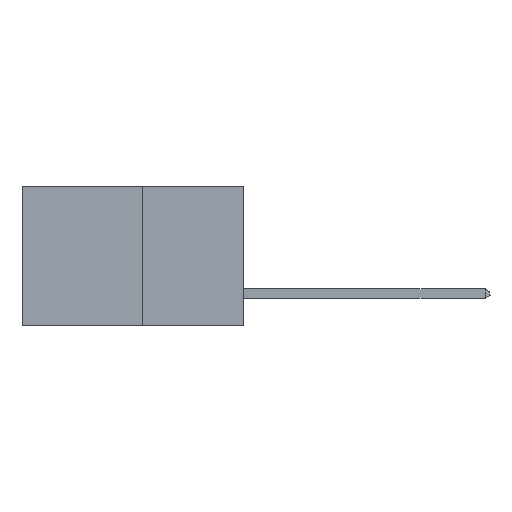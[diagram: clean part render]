
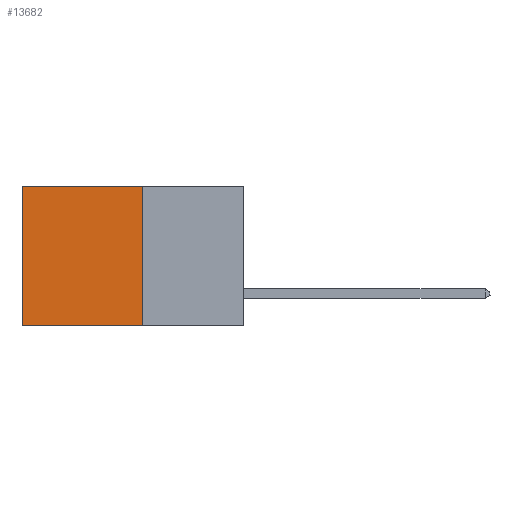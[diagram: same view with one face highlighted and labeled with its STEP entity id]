
A CAD part, left-side view. The second image highlights one B-rep face of the part: STEP entity #13682.
In plain terms, the highlighted planar face has unit normal (-1, 0, 0).
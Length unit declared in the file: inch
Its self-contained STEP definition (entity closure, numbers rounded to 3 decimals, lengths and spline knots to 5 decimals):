
#685 = CARTESIAN_POINT ( 'NONE',  ( 0.277, 0.59, -0.37 ) ) ;
#1333 = VERTEX_POINT ( 'NONE', #685 ) ;
#1390 = EDGE_CURVE ( 'NONE', #10217, #12038, #2702, .T. ) ;
#1473 = AXIS2_PLACEMENT_3D ( 'NONE', #10987, #12049, #5614 ) ;
#1802 = CARTESIAN_POINT ( 'NONE',  ( 0.277, 0.27, -0.37 ) ) ;
#1866 = ORIENTED_EDGE ( 'NONE', *, *, #10497, .T. ) ;
#2213 = ORIENTED_EDGE ( 'NONE', *, *, #12834, .F. ) ;
#2236 = DIRECTION ( 'NONE',  ( 0., 0., -1. ) ) ;
#2417 = CARTESIAN_POINT ( 'NONE',  ( 0.277, 0.27, 0. ) ) ;
#2702 = LINE ( 'NONE', #2417, #13702 ) ;
#3411 = PLANE ( 'NONE',  #1473 ) ;
#4603 = DIRECTION ( 'NONE',  ( 0., 0., -1. ) ) ;
#4695 = EDGE_CURVE ( 'NONE', #10217, #6862, #7697, .T. ) ;
#5614 = DIRECTION ( 'NONE',  ( 0., 0., -1. ) ) ;
#5887 = FACE_OUTER_BOUND ( 'NONE', #12923, .T. ) ;
#6132 = VECTOR ( 'NONE', #2236, 39.37008 ) ;
#6241 = DIRECTION ( 'NONE',  ( 0., 1., 0. ) ) ;
#6554 = CARTESIAN_POINT ( 'NONE',  ( 0.277, 0.59, 0. ) ) ;
#6634 = DIRECTION ( 'NONE',  ( 0., 1., 0. ) ) ;
#6778 = VECTOR ( 'NONE', #6241, 39.37008 ) ;
#6862 = VERTEX_POINT ( 'NONE', #9866 ) ;
#7124 = LINE ( 'NONE', #12607, #6778 ) ;
#7697 = LINE ( 'NONE', #1802, #10844 ) ;
#8892 = ORIENTED_EDGE ( 'NONE', *, *, #4695, .F. ) ;
#9342 = LINE ( 'NONE', #11986, #6132 ) ;
#9866 = CARTESIAN_POINT ( 'NONE',  ( 0.277, 0.27, -0.37 ) ) ;
#10217 = VERTEX_POINT ( 'NONE', #13565 ) ;
#10497 = EDGE_CURVE ( 'NONE', #12038, #1333, #9342, .T. ) ;
#10844 = VECTOR ( 'NONE', #4603, 39.37008 ) ;
#10987 = CARTESIAN_POINT ( 'NONE',  ( 0.277, 0.27, -0.37 ) ) ;
#11986 = CARTESIAN_POINT ( 'NONE',  ( 0.277, 0.59, -0.37 ) ) ;
#12038 = VERTEX_POINT ( 'NONE', #6554 ) ;
#12049 = DIRECTION ( 'NONE',  ( 1., 0., 0. ) ) ;
#12607 = CARTESIAN_POINT ( 'NONE',  ( 0.277, 0.27, -0.37 ) ) ;
#12834 = EDGE_CURVE ( 'NONE', #6862, #1333, #7124, .T. ) ;
#12923 = EDGE_LOOP ( 'NONE', ( #1866, #2213, #8892, #13591 ) ) ;
#13565 = CARTESIAN_POINT ( 'NONE',  ( 0.277, 0.27, 0. ) ) ;
#13591 = ORIENTED_EDGE ( 'NONE', *, *, #1390, .T. ) ;
#13682 = ADVANCED_FACE ( 'NONE', ( #5887 ), #3411, .F. ) ;
#13702 = VECTOR ( 'NONE', #6634, 39.37008 ) ;
